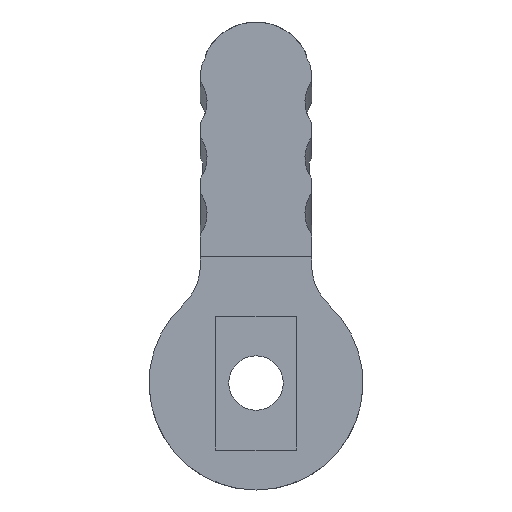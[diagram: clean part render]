
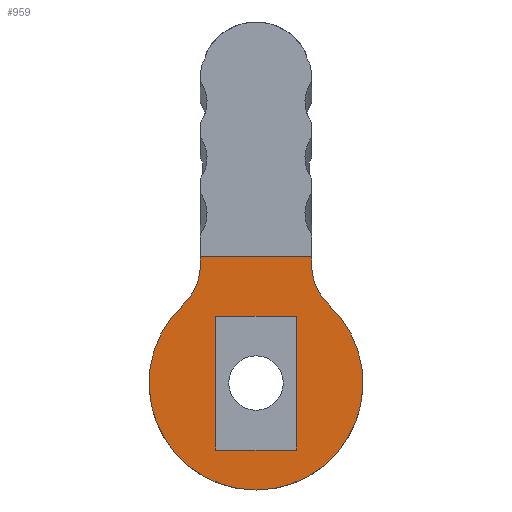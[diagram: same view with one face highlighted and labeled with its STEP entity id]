
A CAD part, front view. The second image highlights one B-rep face of the part: STEP entity #959.
In plain terms, the highlighted planar face has unit normal (0, -1, 0).
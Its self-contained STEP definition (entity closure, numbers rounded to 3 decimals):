
#9 = DIRECTION ( 'NONE',  ( 1., 0., 0. ) ) ;
#39 = CARTESIAN_POINT ( 'NONE',  ( -2.29, 1.79, 3.81 ) ) ;
#47 = EDGE_CURVE ( 'NONE', #826, #1025, #286, .T. ) ;
#126 = DIRECTION ( 'NONE',  ( 0., -1., 0. ) ) ;
#136 = VERTEX_POINT ( 'NONE', #1701 ) ;
#142 = DIRECTION ( 'NONE',  ( 0., 1., 0. ) ) ;
#149 = EDGE_CURVE ( 'NONE', #1568, #338, #1795, .T. ) ;
#191 = CARTESIAN_POINT ( 'NONE',  ( 3.16, 1.79, 7.19 ) ) ;
#235 = VECTOR ( 'NONE', #2024, 1000. ) ;
#248 = CARTESIAN_POINT ( 'NONE',  ( 0., 1.79, 0. ) ) ;
#286 = LINE ( 'NONE', #1026, #235 ) ;
#312 = ORIENTED_EDGE ( 'NONE', *, *, #686, .T. ) ;
#325 = CARTESIAN_POINT ( 'NONE',  ( 3.16, 1.79, 6.747 ) ) ;
#338 = VERTEX_POINT ( 'NONE', #2000 ) ;
#341 = ORIENTED_EDGE ( 'NONE', *, *, #1951, .T. ) ;
#375 = EDGE_CURVE ( 'NONE', #500, #423, #943, .T. ) ;
#410 = DIRECTION ( 'NONE',  ( 0., 0., 1. ) ) ;
#414 = VECTOR ( 'NONE', #9, 1000. ) ;
#415 = DIRECTION ( 'NONE',  ( 0., 0., 1. ) ) ;
#423 = VERTEX_POINT ( 'NONE', #1499 ) ;
#435 = DIRECTION ( 'NONE',  ( 0., 0., -1. ) ) ;
#486 = DIRECTION ( 'NONE',  ( 0., 0., 1. ) ) ;
#500 = VERTEX_POINT ( 'NONE', #1858 ) ;
#516 = LINE ( 'NONE', #191, #414 ) ;
#567 = CARTESIAN_POINT ( 'NONE',  ( 6.32, 1.79, 6.747 ) ) ;
#572 = AXIS2_PLACEMENT_3D ( 'NONE', #802, #1805, #812 ) ;
#593 = CIRCLE ( 'NONE', #1971, 6.085 ) ;
#611 = VECTOR ( 'NONE', #486, 1000. ) ;
#637 = PLANE ( 'NONE',  #572 ) ;
#639 = EDGE_CURVE ( 'NONE', #136, #1278, #516, .T. ) ;
#647 = LINE ( 'NONE', #1241, #1472 ) ;
#667 = CIRCLE ( 'NONE', #1715, 6.085 ) ;
#675 = CARTESIAN_POINT ( 'NONE',  ( -2.29, 1.79, -3.81 ) ) ;
#686 = EDGE_CURVE ( 'NONE', #1636, #1565, #1588, .T. ) ;
#753 = DIRECTION ( 'NONE',  ( 0., 0., -1. ) ) ;
#785 = FACE_BOUND ( 'NONE', #1620, .T. ) ;
#787 = CARTESIAN_POINT ( 'NONE',  ( 0., 1.79, -6.085 ) ) ;
#789 = ORIENTED_EDGE ( 'NONE', *, *, #1968, .F. ) ;
#802 = CARTESIAN_POINT ( 'NONE',  ( 0., 1.79, 17.385 ) ) ;
#812 = DIRECTION ( 'NONE',  ( 0., 0., 1. ) ) ;
#819 = ORIENTED_EDGE ( 'NONE', *, *, #1515, .F. ) ;
#826 = VERTEX_POINT ( 'NONE', #1587 ) ;
#846 = ORIENTED_EDGE ( 'NONE', *, *, #639, .F. ) ;
#848 = ORIENTED_EDGE ( 'NONE', *, *, #375, .F. ) ;
#879 = VECTOR ( 'NONE', #435, 1000. ) ;
#902 = AXIS2_PLACEMENT_3D ( 'NONE', #567, #1740, #753 ) ;
#943 = CIRCLE ( 'NONE', #1296, 3.16 ) ;
#959 = ADVANCED_FACE ( 'NONE', ( #1222, #785 ), #637, .F. ) ;
#1009 = VECTOR ( 'NONE', #1317, 1000. ) ;
#1012 = CARTESIAN_POINT ( 'NONE',  ( -6.32, 1.79, 6.747 ) ) ;
#1025 = VERTEX_POINT ( 'NONE', #675 ) ;
#1026 = CARTESIAN_POINT ( 'NONE',  ( -2.29, 1.79, -3.81 ) ) ;
#1055 = DIRECTION ( 'NONE',  ( 1., 0., 0. ) ) ;
#1106 = CARTESIAN_POINT ( 'NONE',  ( 2.29, 1.79, -3.81 ) ) ;
#1142 = CARTESIAN_POINT ( 'NONE',  ( 0., 1.79, 0. ) ) ;
#1154 = CARTESIAN_POINT ( 'NONE',  ( -3.16, 1.79, 17.385 ) ) ;
#1214 = LINE ( 'NONE', #1106, #879 ) ;
#1222 = FACE_OUTER_BOUND ( 'NONE', #1601, .T. ) ;
#1237 = ORIENTED_EDGE ( 'NONE', *, *, #1360, .T. ) ;
#1241 = CARTESIAN_POINT ( 'NONE',  ( -2.29, 1.79, -3.81 ) ) ;
#1257 = ORIENTED_EDGE ( 'NONE', *, *, #149, .F. ) ;
#1278 = VERTEX_POINT ( 'NONE', #1571 ) ;
#1296 = AXIS2_PLACEMENT_3D ( 'NONE', #1012, #126, #1375 ) ;
#1307 = DIRECTION ( 'NONE',  ( 0., 0., 1. ) ) ;
#1317 = DIRECTION ( 'NONE',  ( 0., 0., -1. ) ) ;
#1360 = EDGE_CURVE ( 'NONE', #1565, #826, #1214, .T. ) ;
#1375 = DIRECTION ( 'NONE',  ( 0., 0., 1. ) ) ;
#1409 = DIRECTION ( 'NONE',  ( 0., 1., 0. ) ) ;
#1440 = LINE ( 'NONE', #1154, #611 ) ;
#1472 = VECTOR ( 'NONE', #410, 1000. ) ;
#1487 = EDGE_CURVE ( 'NONE', #338, #2072, #667, .T. ) ;
#1499 = CARTESIAN_POINT ( 'NONE',  ( -3.16, 1.79, 6.747 ) ) ;
#1505 = CARTESIAN_POINT ( 'NONE',  ( -2.29, 1.79, 3.81 ) ) ;
#1515 = EDGE_CURVE ( 'NONE', #1278, #1568, #2109, .T. ) ;
#1525 = EDGE_CURVE ( 'NONE', #423, #136, #1440, .T. ) ;
#1565 = VERTEX_POINT ( 'NONE', #2159 ) ;
#1568 = VERTEX_POINT ( 'NONE', #325 ) ;
#1571 = CARTESIAN_POINT ( 'NONE',  ( 3.16, 1.79, 7.19 ) ) ;
#1587 = CARTESIAN_POINT ( 'NONE',  ( 2.29, 1.79, -3.81 ) ) ;
#1588 = LINE ( 'NONE', #39, #2032 ) ;
#1601 = EDGE_LOOP ( 'NONE', ( #819, #846, #1673, #848, #789, #1648, #1257 ) ) ;
#1620 = EDGE_LOOP ( 'NONE', ( #312, #1237, #1670, #341 ) ) ;
#1636 = VERTEX_POINT ( 'NONE', #1505 ) ;
#1637 = CARTESIAN_POINT ( 'NONE',  ( 3.16, 1.79, 17.385 ) ) ;
#1648 = ORIENTED_EDGE ( 'NONE', *, *, #1487, .F. ) ;
#1670 = ORIENTED_EDGE ( 'NONE', *, *, #47, .T. ) ;
#1673 = ORIENTED_EDGE ( 'NONE', *, *, #1525, .F. ) ;
#1701 = CARTESIAN_POINT ( 'NONE',  ( -3.16, 1.79, 7.19 ) ) ;
#1715 = AXIS2_PLACEMENT_3D ( 'NONE', #1142, #142, #1307 ) ;
#1740 = DIRECTION ( 'NONE',  ( 0., -1., 0. ) ) ;
#1795 = CIRCLE ( 'NONE', #902, 3.16 ) ;
#1805 = DIRECTION ( 'NONE',  ( 0., 1., 0. ) ) ;
#1858 = CARTESIAN_POINT ( 'NONE',  ( -4.16, 1.79, 4.441 ) ) ;
#1951 = EDGE_CURVE ( 'NONE', #1025, #1636, #647, .T. ) ;
#1968 = EDGE_CURVE ( 'NONE', #2072, #500, #593, .T. ) ;
#1971 = AXIS2_PLACEMENT_3D ( 'NONE', #248, #1409, #415 ) ;
#2000 = CARTESIAN_POINT ( 'NONE',  ( 4.16, 1.79, 4.441 ) ) ;
#2024 = DIRECTION ( 'NONE',  ( -1., 0., 0. ) ) ;
#2032 = VECTOR ( 'NONE', #1055, 1000. ) ;
#2072 = VERTEX_POINT ( 'NONE', #787 ) ;
#2109 = LINE ( 'NONE', #1637, #1009 ) ;
#2159 = CARTESIAN_POINT ( 'NONE',  ( 2.29, 1.79, 3.81 ) ) ;
